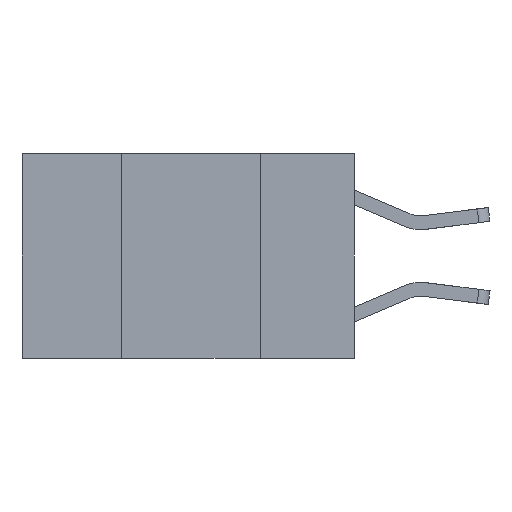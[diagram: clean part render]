
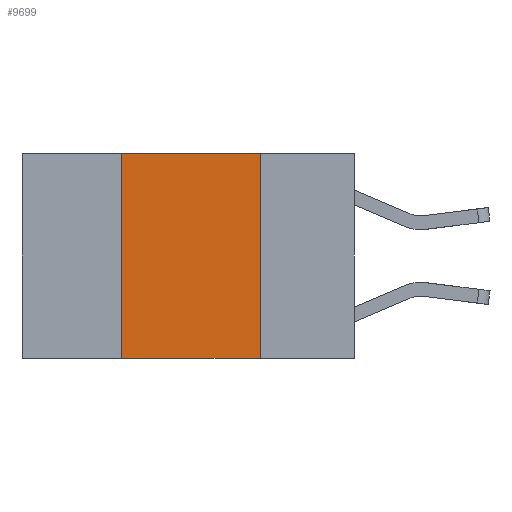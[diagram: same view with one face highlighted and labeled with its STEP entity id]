
A CAD part, left-side view. The second image highlights one B-rep face of the part: STEP entity #9699.
In plain terms, the highlighted planar face has unit normal (-1, 0, 0).
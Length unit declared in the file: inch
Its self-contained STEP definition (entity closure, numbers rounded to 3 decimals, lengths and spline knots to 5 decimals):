
#1 = ORIENTED_EDGE ( 'NONE', *, *, #943, .T. ) ;
#463 = VERTEX_POINT ( 'NONE', #8969 ) ;
#491 = CARTESIAN_POINT ( 'NONE',  ( 0., 0.17, 0. ) ) ;
#739 = VERTEX_POINT ( 'NONE', #7359 ) ;
#772 = VECTOR ( 'NONE', #10843, 39.37008 ) ;
#943 = EDGE_CURVE ( 'NONE', #5669, #739, #10214, .T. ) ;
#1021 = VERTEX_POINT ( 'NONE', #1939 ) ;
#1502 = LINE ( 'NONE', #8958, #772 ) ;
#1691 = DIRECTION ( 'NONE',  ( 0., -1., 0. ) ) ;
#1700 = DIRECTION ( 'NONE',  ( 0., 0., -1. ) ) ;
#1762 = PLANE ( 'NONE',  #8563 ) ;
#1939 = CARTESIAN_POINT ( 'NONE',  ( 0., 0.17, 0. ) ) ;
#1998 = EDGE_CURVE ( 'NONE', #1021, #739, #9031, .T. ) ;
#2498 = VECTOR ( 'NONE', #1691, 39.37008 ) ;
#2591 = VECTOR ( 'NONE', #9963, 39.37008 ) ;
#3227 = VECTOR ( 'NONE', #1700, 39.37008 ) ;
#3462 = DIRECTION ( 'NONE',  ( 0., 0., -1. ) ) ;
#5669 = VERTEX_POINT ( 'NONE', #7516 ) ;
#5784 = ORIENTED_EDGE ( 'NONE', *, *, #1998, .F. ) ;
#6198 = LINE ( 'NONE', #8713, #2591 ) ;
#6301 = EDGE_CURVE ( 'NONE', #463, #1021, #1502, .T. ) ;
#6446 = FACE_OUTER_BOUND ( 'NONE', #7273, .T. ) ;
#7273 = EDGE_LOOP ( 'NONE', ( #5784, #11990, #9648, #1 ) ) ;
#7308 = CARTESIAN_POINT ( 'NONE',  ( 0., 0.6, 0. ) ) ;
#7359 = CARTESIAN_POINT ( 'NONE',  ( 0., 0.17, -0.37 ) ) ;
#7516 = CARTESIAN_POINT ( 'NONE',  ( 0., 0.42, -0.37 ) ) ;
#8563 = AXIS2_PLACEMENT_3D ( 'NONE', #7308, #11143, #3462 ) ;
#8713 = CARTESIAN_POINT ( 'NONE',  ( 0., 0.42, 0. ) ) ;
#8958 = CARTESIAN_POINT ( 'NONE',  ( 0., 0.6, 0. ) ) ;
#8969 = CARTESIAN_POINT ( 'NONE',  ( 0., 0.42, 0. ) ) ;
#9031 = LINE ( 'NONE', #491, #3227 ) ;
#9334 = CARTESIAN_POINT ( 'NONE',  ( 0., 0.6, -0.37 ) ) ;
#9648 = ORIENTED_EDGE ( 'NONE', *, *, #10941, .F. ) ;
#9699 = ADVANCED_FACE ( 'NONE', ( #6446 ), #1762, .F. ) ;
#9963 = DIRECTION ( 'NONE',  ( 0., 0., 1. ) ) ;
#10214 = LINE ( 'NONE', #9334, #2498 ) ;
#10843 = DIRECTION ( 'NONE',  ( 0., -1., 0. ) ) ;
#10941 = EDGE_CURVE ( 'NONE', #5669, #463, #6198, .T. ) ;
#11143 = DIRECTION ( 'NONE',  ( 1., 0., 0. ) ) ;
#11990 = ORIENTED_EDGE ( 'NONE', *, *, #6301, .F. ) ;
